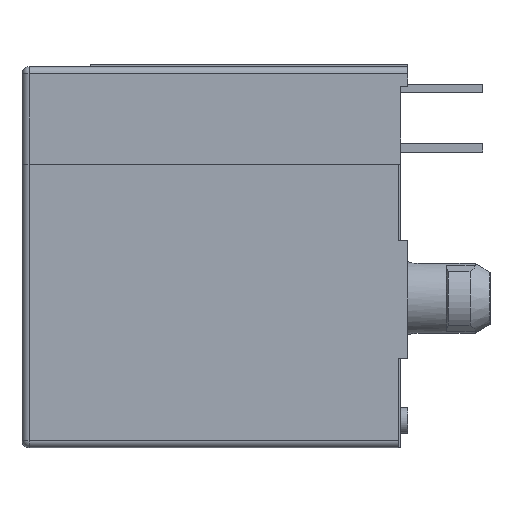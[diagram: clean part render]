
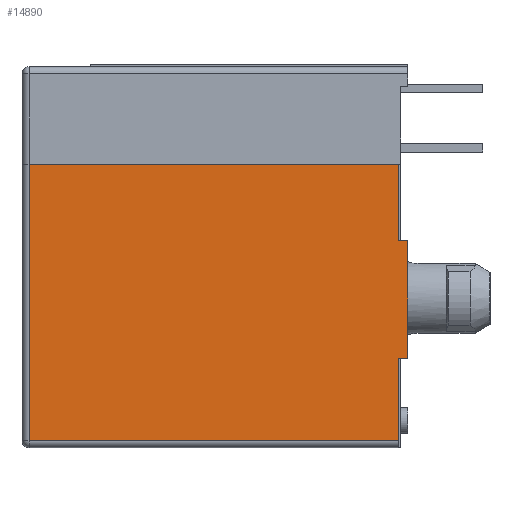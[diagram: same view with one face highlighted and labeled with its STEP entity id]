
A CAD part, left-side view. The second image highlights one B-rep face of the part: STEP entity #14890.
In plain terms, the highlighted planar face has unit normal (-1, 0, 0).
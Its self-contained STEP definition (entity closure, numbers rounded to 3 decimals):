
#39 = ORIENTED_EDGE ( 'NONE', *, *, #21151, .T. ) ;
#125 = CARTESIAN_POINT ( 'NONE',  ( -7.7, -16., -2.55 ) ) ;
#924 = CARTESIAN_POINT ( 'NONE',  ( -7.7, 0., 5.7 ) ) ;
#1048 = VERTEX_POINT ( 'NONE', #12647 ) ;
#1382 = VECTOR ( 'NONE', #8708, 1000. ) ;
#1980 = EDGE_CURVE ( 'NONE', #3168, #1985, #11170, .T. ) ;
#1985 = VERTEX_POINT ( 'NONE', #7247 ) ;
#2059 = CARTESIAN_POINT ( 'NONE',  ( -7.7, -16.4, 5.7 ) ) ;
#2297 = VERTEX_POINT ( 'NONE', #11514 ) ;
#3168 = VERTEX_POINT ( 'NONE', #10965 ) ;
#3438 = EDGE_CURVE ( 'NONE', #18676, #8734, #8250, .T. ) ;
#3535 = EDGE_CURVE ( 'NONE', #1048, #2297, #7672, .T. ) ;
#4457 = CARTESIAN_POINT ( 'NONE',  ( -7.7, -16., 2.45 ) ) ;
#4881 = LINE ( 'NONE', #15986, #16251 ) ;
#5465 = LINE ( 'NONE', #6693, #1382 ) ;
#5521 = ORIENTED_EDGE ( 'NONE', *, *, #23841, .T. ) ;
#5583 = DIRECTION ( 'NONE',  ( 0., 0., 1. ) ) ;
#5935 = CARTESIAN_POINT ( 'NONE',  ( -7.7, -16.1, -2.55 ) ) ;
#6245 = VECTOR ( 'NONE', #14090, 1000. ) ;
#6271 = VERTEX_POINT ( 'NONE', #12564 ) ;
#6398 = ORIENTED_EDGE ( 'NONE', *, *, #1980, .T. ) ;
#6425 = DIRECTION ( 'NONE',  ( 0., -1., 0. ) ) ;
#6693 = CARTESIAN_POINT ( 'NONE',  ( -7.7, -16., 5.7 ) ) ;
#7247 = CARTESIAN_POINT ( 'NONE',  ( -7.7, -0.3, -6.05 ) ) ;
#7672 = LINE ( 'NONE', #4457, #9084 ) ;
#8250 = LINE ( 'NONE', #5935, #22282 ) ;
#8456 = ORIENTED_EDGE ( 'NONE', *, *, #3535, .F. ) ;
#8708 = DIRECTION ( 'NONE',  ( 0., 0., 1. ) ) ;
#8734 = VERTEX_POINT ( 'NONE', #15387 ) ;
#9044 = FACE_OUTER_BOUND ( 'NONE', #24172, .T. ) ;
#9084 = VECTOR ( 'NONE', #6425, 1000. ) ;
#9444 = CARTESIAN_POINT ( 'NONE',  ( -7.7, -16., -6.05 ) ) ;
#10209 = CARTESIAN_POINT ( 'NONE',  ( -7.7, 0., 5.7 ) ) ;
#10410 = LINE ( 'NONE', #10209, #13367 ) ;
#10674 = ORIENTED_EDGE ( 'NONE', *, *, #12223, .F. ) ;
#10965 = CARTESIAN_POINT ( 'NONE',  ( -7.7, -0.3, 5.7 ) ) ;
#11136 = LINE ( 'NONE', #22493, #14095 ) ;
#11170 = LINE ( 'NONE', #17854, #6245 ) ;
#11514 = CARTESIAN_POINT ( 'NONE',  ( -7.7, -16.4, 2.45 ) ) ;
#11522 = DIRECTION ( 'NONE',  ( 0., -1., 0. ) ) ;
#11774 = DIRECTION ( 'NONE',  ( 0., 1., 0. ) ) ;
#12073 = EDGE_CURVE ( 'NONE', #1048, #6271, #5465, .T. ) ;
#12223 = EDGE_CURVE ( 'NONE', #23825, #1985, #4881, .T. ) ;
#12564 = CARTESIAN_POINT ( 'NONE',  ( -7.7, -16., 5.7 ) ) ;
#12647 = CARTESIAN_POINT ( 'NONE',  ( -7.7, -16., 2.45 ) ) ;
#13367 = VECTOR ( 'NONE', #11774, 1000. ) ;
#14090 = DIRECTION ( 'NONE',  ( 0., 0., -1. ) ) ;
#14095 = VECTOR ( 'NONE', #5583, 1000. ) ;
#14199 = PLANE ( 'NONE',  #22679 ) ;
#14890 = ADVANCED_FACE ( 'NONE', ( #9044 ), #14199, .T. ) ;
#15027 = ORIENTED_EDGE ( 'NONE', *, *, #12073, .T. ) ;
#15387 = CARTESIAN_POINT ( 'NONE',  ( -7.7, -16.4, -2.55 ) ) ;
#15693 = LINE ( 'NONE', #2059, #17729 ) ;
#15986 = CARTESIAN_POINT ( 'NONE',  ( -7.7, -16.147, -6.05 ) ) ;
#16070 = EDGE_CURVE ( 'NONE', #6271, #3168, #10410, .T. ) ;
#16251 = VECTOR ( 'NONE', #23807, 1000. ) ;
#16989 = DIRECTION ( 'NONE',  ( 0., 0., 1. ) ) ;
#17729 = VECTOR ( 'NONE', #16989, 1000. ) ;
#17854 = CARTESIAN_POINT ( 'NONE',  ( -7.7, -0.3, 5.7 ) ) ;
#18676 = VERTEX_POINT ( 'NONE', #125 ) ;
#19665 = DIRECTION ( 'NONE',  ( 0., 0., -1. ) ) ;
#21072 = ORIENTED_EDGE ( 'NONE', *, *, #3438, .T. ) ;
#21151 = EDGE_CURVE ( 'NONE', #23825, #18676, #11136, .T. ) ;
#22282 = VECTOR ( 'NONE', #11522, 1000. ) ;
#22493 = CARTESIAN_POINT ( 'NONE',  ( -7.7, -16., 5.7 ) ) ;
#22679 = AXIS2_PLACEMENT_3D ( 'NONE', #924, #23439, #19665 ) ;
#23082 = ORIENTED_EDGE ( 'NONE', *, *, #16070, .T. ) ;
#23439 = DIRECTION ( 'NONE',  ( -1., 0., 0. ) ) ;
#23807 = DIRECTION ( 'NONE',  ( 0., 1., 0. ) ) ;
#23825 = VERTEX_POINT ( 'NONE', #9444 ) ;
#23841 = EDGE_CURVE ( 'NONE', #8734, #2297, #15693, .T. ) ;
#24172 = EDGE_LOOP ( 'NONE', ( #8456, #15027, #23082, #6398, #10674, #39, #21072, #5521 ) ) ;
